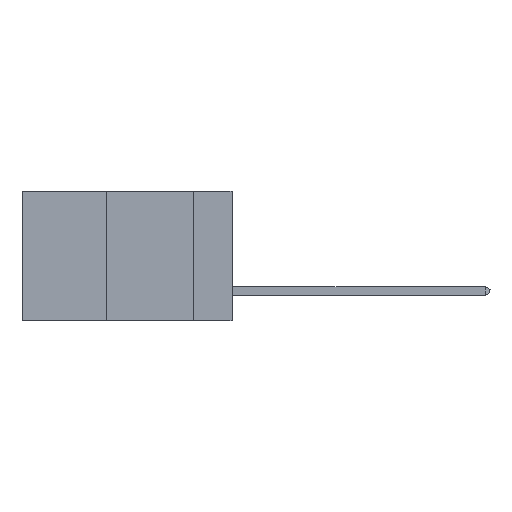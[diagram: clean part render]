
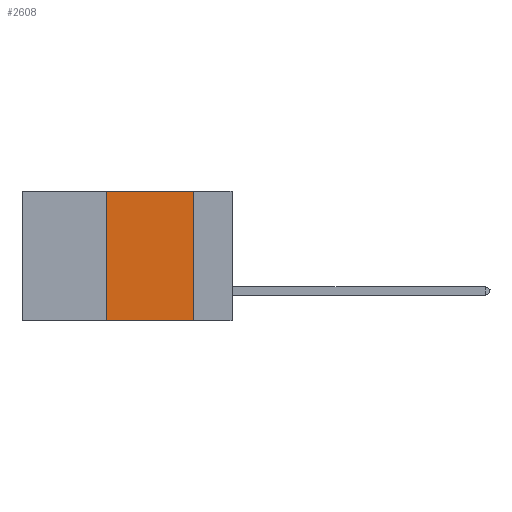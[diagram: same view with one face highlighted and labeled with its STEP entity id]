
A CAD part, left-side view. The second image highlights one B-rep face of the part: STEP entity #2608.
In plain terms, the highlighted planar face has unit normal (-1, 0, 0).
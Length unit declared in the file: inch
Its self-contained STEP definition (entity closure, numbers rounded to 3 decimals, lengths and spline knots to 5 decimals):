
#869 = LINE ( 'NONE', #6917, #2157 ) ;
#1048 = PLANE ( 'NONE',  #3824 ) ;
#1862 = DIRECTION ( 'NONE',  ( 1., 0., 0. ) ) ;
#2157 = VECTOR ( 'NONE', #7748, 39.37008 ) ;
#2608 = ADVANCED_FACE ( 'NONE', ( #8559 ), #1048, .F. ) ;
#2655 = VECTOR ( 'NONE', #4897, 39.37008 ) ;
#2981 = CARTESIAN_POINT ( 'NONE',  ( 0., 0.6, 0. ) ) ;
#3038 = VERTEX_POINT ( 'NONE', #10178 ) ;
#3063 = LINE ( 'NONE', #8145, #6592 ) ;
#3270 = DIRECTION ( 'NONE',  ( 0., 0., -1. ) ) ;
#3310 = DIRECTION ( 'NONE',  ( 0., 0., -1. ) ) ;
#3521 = EDGE_CURVE ( 'NONE', #8015, #7248, #3063, .T. ) ;
#3557 = EDGE_CURVE ( 'NONE', #6751, #7248, #8665, .T. ) ;
#3824 = AXIS2_PLACEMENT_3D ( 'NONE', #6692, #1862, #3310 ) ;
#4265 = EDGE_CURVE ( 'NONE', #6751, #3038, #869, .T. ) ;
#4865 = CARTESIAN_POINT ( 'NONE',  ( 0., 0.11, 0. ) ) ;
#4897 = DIRECTION ( 'NONE',  ( 0., -1., 0. ) ) ;
#5473 = EDGE_LOOP ( 'NONE', ( #7294, #10351, #5493, #6462 ) ) ;
#5493 = ORIENTED_EDGE ( 'NONE', *, *, #4265, .F. ) ;
#6126 = CARTESIAN_POINT ( 'NONE',  ( 0., 0.36, -0.37 ) ) ;
#6462 = ORIENTED_EDGE ( 'NONE', *, *, #3557, .T. ) ;
#6592 = VECTOR ( 'NONE', #3270, 39.37008 ) ;
#6692 = CARTESIAN_POINT ( 'NONE',  ( 0., 0.6, 0. ) ) ;
#6751 = VERTEX_POINT ( 'NONE', #6126 ) ;
#6917 = CARTESIAN_POINT ( 'NONE',  ( 0., 0.36, 0. ) ) ;
#7027 = LINE ( 'NONE', #2981, #9440 ) ;
#7248 = VERTEX_POINT ( 'NONE', #10103 ) ;
#7294 = ORIENTED_EDGE ( 'NONE', *, *, #3521, .F. ) ;
#7339 = EDGE_CURVE ( 'NONE', #3038, #8015, #7027, .T. ) ;
#7385 = CARTESIAN_POINT ( 'NONE',  ( 0., 0.6, -0.37 ) ) ;
#7748 = DIRECTION ( 'NONE',  ( 0., 0., 1. ) ) ;
#8015 = VERTEX_POINT ( 'NONE', #4865 ) ;
#8145 = CARTESIAN_POINT ( 'NONE',  ( 0., 0.11, 0. ) ) ;
#8559 = FACE_OUTER_BOUND ( 'NONE', #5473, .T. ) ;
#8665 = LINE ( 'NONE', #7385, #2655 ) ;
#9440 = VECTOR ( 'NONE', #10457, 39.37008 ) ;
#10103 = CARTESIAN_POINT ( 'NONE',  ( 0., 0.11, -0.37 ) ) ;
#10178 = CARTESIAN_POINT ( 'NONE',  ( 0., 0.36, 0. ) ) ;
#10351 = ORIENTED_EDGE ( 'NONE', *, *, #7339, .F. ) ;
#10457 = DIRECTION ( 'NONE',  ( 0., -1., 0. ) ) ;
